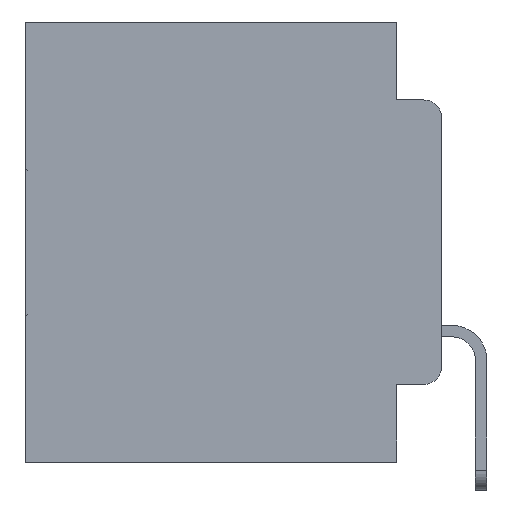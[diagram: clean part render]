
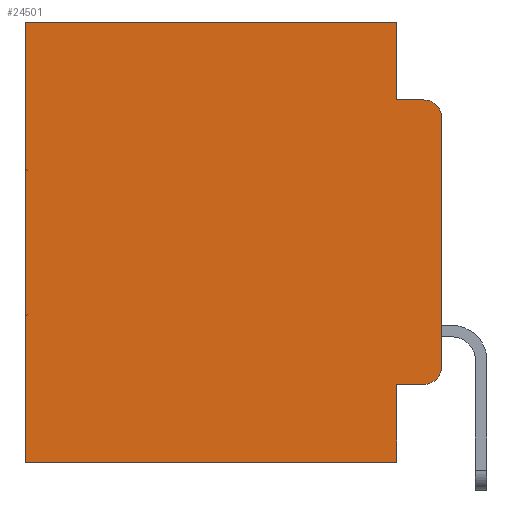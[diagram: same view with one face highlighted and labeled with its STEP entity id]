
A CAD part, left-side view. The second image highlights one B-rep face of the part: STEP entity #24501.
In plain terms, the highlighted planar face has unit normal (-1, 0, 0).
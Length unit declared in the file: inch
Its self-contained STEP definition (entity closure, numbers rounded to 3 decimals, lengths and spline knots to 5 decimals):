
#218 = VERTEX_POINT ( 'NONE', #25674 ) ;
#395 = ORIENTED_EDGE ( 'NONE', *, *, #31190, .T. ) ;
#917 = ORIENTED_EDGE ( 'NONE', *, *, #1913, .F. ) ;
#1913 = EDGE_CURVE ( 'NONE', #12299, #22366, #22583, .T. ) ;
#2809 = CARTESIAN_POINT ( 'NONE',  ( 0.298, 0.473, 0. ) ) ;
#3572 = ORIENTED_EDGE ( 'NONE', *, *, #9032, .T. ) ;
#3650 = CARTESIAN_POINT ( 'NONE',  ( 0.298, 0., -0.5 ) ) ;
#3674 = EDGE_CURVE ( 'NONE', #21039, #12299, #16716, .T. ) ;
#3960 = CARTESIAN_POINT ( 'NONE',  ( 0.298, 0.051, -0.5 ) ) ;
#4097 = ORIENTED_EDGE ( 'NONE', *, *, #3674, .F. ) ;
#4185 = ORIENTED_EDGE ( 'NONE', *, *, #27915, .T. ) ;
#4244 = LINE ( 'NONE', #29644, #28980 ) ;
#4953 = LINE ( 'NONE', #19136, #22897 ) ;
#5434 = ORIENTED_EDGE ( 'NONE', *, *, #21819, .T. ) ;
#5589 = CARTESIAN_POINT ( 'NONE',  ( 0.298, 0.051, -0.0885 ) ) ;
#6819 = ORIENTED_EDGE ( 'NONE', *, *, #12895, .F. ) ;
#7093 = CARTESIAN_POINT ( 'NONE',  ( 0.298, 0.02, -0.3915 ) ) ;
#8253 = LINE ( 'NONE', #2809, #20296 ) ;
#8846 = EDGE_LOOP ( 'NONE', ( #6819, #22990, #917, #4097, #395, #3572, #18075, #10520, #5434, #4185 ) ) ;
#8907 = DIRECTION ( 'NONE',  ( 0., 1., 0. ) ) ;
#9032 = EDGE_CURVE ( 'NONE', #30833, #218, #8253, .T. ) ;
#9357 = VERTEX_POINT ( 'NONE', #19081 ) ;
#9615 = DIRECTION ( 'NONE',  ( 0., 0., -1. ) ) ;
#9650 = DIRECTION ( 'NONE',  ( 0., 0., -1. ) ) ;
#9714 = CARTESIAN_POINT ( 'NONE',  ( 0.298, 0.051, -0.4115 ) ) ;
#10187 = VECTOR ( 'NONE', #13218, 39.37008 ) ;
#10520 = ORIENTED_EDGE ( 'NONE', *, *, #10673, .F. ) ;
#10673 = EDGE_CURVE ( 'NONE', #26597, #21784, #31080, .T. ) ;
#10727 = CARTESIAN_POINT ( 'NONE',  ( 0.298, 0., 0. ) ) ;
#10855 = DIRECTION ( 'NONE',  ( -1., 0., 0. ) ) ;
#11167 = AXIS2_PLACEMENT_3D ( 'NONE', #7093, #23895, #9650 ) ;
#11837 = CARTESIAN_POINT ( 'NONE',  ( 0.298, 0.02, -0.0885 ) ) ;
#12299 = VERTEX_POINT ( 'NONE', #5589 ) ;
#12895 = EDGE_CURVE ( 'NONE', #15095, #25877, #28412, .T. ) ;
#13218 = DIRECTION ( 'NONE',  ( 0., 0., -1. ) ) ;
#15095 = VERTEX_POINT ( 'NONE', #19941 ) ;
#16221 = EDGE_CURVE ( 'NONE', #15095, #22366, #16773, .T. ) ;
#16392 = VECTOR ( 'NONE', #8907, 39.37008 ) ;
#16716 = LINE ( 'NONE', #29400, #10187 ) ;
#16773 = CIRCLE ( 'NONE', #25864, 0.02 ) ;
#17139 = LINE ( 'NONE', #3650, #16392 ) ;
#17395 = EDGE_CURVE ( 'NONE', #21784, #218, #17139, .T. ) ;
#17521 = DIRECTION ( 'NONE',  ( 0., -1., 0. ) ) ;
#18075 = ORIENTED_EDGE ( 'NONE', *, *, #17395, .F. ) ;
#19081 = CARTESIAN_POINT ( 'NONE',  ( 0.298, 0.02, -0.4115 ) ) ;
#19136 = CARTESIAN_POINT ( 'NONE',  ( 0.298, 0.051, -0.4115 ) ) ;
#19941 = CARTESIAN_POINT ( 'NONE',  ( 0.298, 0., -0.1085 ) ) ;
#20140 = CARTESIAN_POINT ( 'NONE',  ( 0.298, 0.051, 0. ) ) ;
#20205 = DIRECTION ( 'NONE',  ( 0., 0., -1. ) ) ;
#20296 = VECTOR ( 'NONE', #20205, 39.37008 ) ;
#20513 = CARTESIAN_POINT ( 'NONE',  ( 0.298, 0.051, -0.0885 ) ) ;
#21039 = VERTEX_POINT ( 'NONE', #21044 ) ;
#21044 = CARTESIAN_POINT ( 'NONE',  ( 0.298, 0.051, 0. ) ) ;
#21425 = CARTESIAN_POINT ( 'NONE',  ( 0.298, 0., -0.3915 ) ) ;
#21492 = PLANE ( 'NONE',  #26162 ) ;
#21672 = CARTESIAN_POINT ( 'NONE',  ( 0.298, 0.473, 0. ) ) ;
#21784 = VERTEX_POINT ( 'NONE', #3960 ) ;
#21819 = EDGE_CURVE ( 'NONE', #26597, #9357, #4953, .T. ) ;
#21829 = VECTOR ( 'NONE', #17521, 39.37008 ) ;
#22366 = VERTEX_POINT ( 'NONE', #11837 ) ;
#22422 = DIRECTION ( 'NONE',  ( 0., 0., -1. ) ) ;
#22583 = LINE ( 'NONE', #20513, #21829 ) ;
#22897 = VECTOR ( 'NONE', #28173, 39.37008 ) ;
#22990 = ORIENTED_EDGE ( 'NONE', *, *, #16221, .T. ) ;
#23135 = VECTOR ( 'NONE', #24901, 39.37008 ) ;
#23151 = CIRCLE ( 'NONE', #11167, 0.02 ) ;
#23858 = DIRECTION ( 'NONE',  ( 1., 0., 0. ) ) ;
#23895 = DIRECTION ( 'NONE',  ( -1., 0., 0. ) ) ;
#24501 = ADVANCED_FACE ( 'NONE', ( #25914 ), #21492, .F. ) ;
#24534 = VECTOR ( 'NONE', #22422, 39.37008 ) ;
#24901 = DIRECTION ( 'NONE',  ( 0., 0., -1. ) ) ;
#25033 = CARTESIAN_POINT ( 'NONE',  ( 0.298, 0.02, -0.1085 ) ) ;
#25674 = CARTESIAN_POINT ( 'NONE',  ( 0.298, 0.473, -0.5 ) ) ;
#25864 = AXIS2_PLACEMENT_3D ( 'NONE', #25033, #10855, #27258 ) ;
#25877 = VERTEX_POINT ( 'NONE', #21425 ) ;
#25914 = FACE_OUTER_BOUND ( 'NONE', #8846, .T. ) ;
#26162 = AXIS2_PLACEMENT_3D ( 'NONE', #28258, #23858, #9615 ) ;
#26597 = VERTEX_POINT ( 'NONE', #9714 ) ;
#27258 = DIRECTION ( 'NONE',  ( 0., 0., -1. ) ) ;
#27431 = DIRECTION ( 'NONE',  ( 0., 1., 0. ) ) ;
#27915 = EDGE_CURVE ( 'NONE', #9357, #25877, #23151, .T. ) ;
#28173 = DIRECTION ( 'NONE',  ( 0., -1., 0. ) ) ;
#28258 = CARTESIAN_POINT ( 'NONE',  ( 0.298, 0., 0. ) ) ;
#28412 = LINE ( 'NONE', #10727, #23135 ) ;
#28980 = VECTOR ( 'NONE', #27431, 39.37008 ) ;
#29400 = CARTESIAN_POINT ( 'NONE',  ( 0.298, 0.051, 0. ) ) ;
#29644 = CARTESIAN_POINT ( 'NONE',  ( 0.298, 0., 0. ) ) ;
#30833 = VERTEX_POINT ( 'NONE', #21672 ) ;
#31080 = LINE ( 'NONE', #20140, #24534 ) ;
#31190 = EDGE_CURVE ( 'NONE', #21039, #30833, #4244, .T. ) ;
